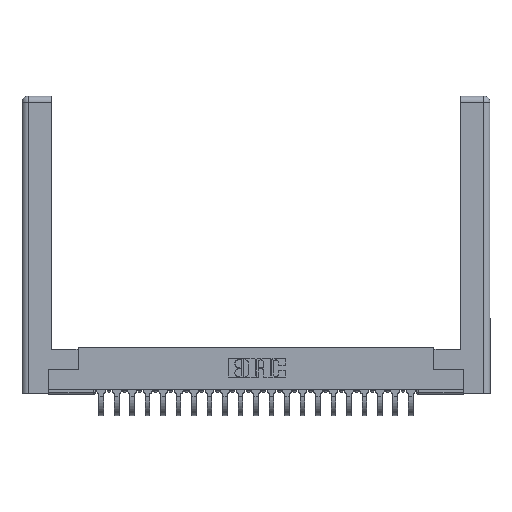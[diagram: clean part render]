
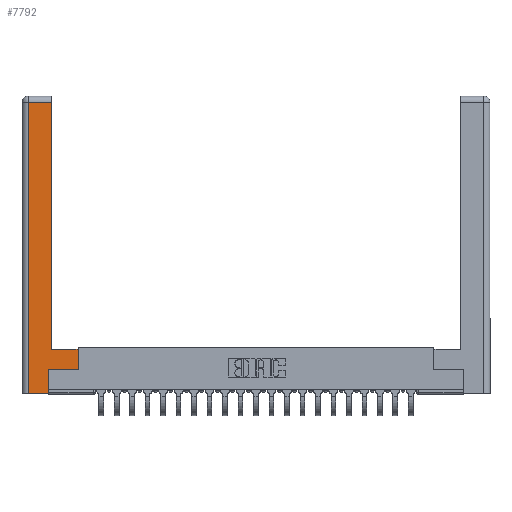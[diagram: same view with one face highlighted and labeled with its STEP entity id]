
A CAD part, top view. The second image highlights one B-rep face of the part: STEP entity #7792.
In plain terms, the highlighted planar face has unit normal (0, 0, 1).
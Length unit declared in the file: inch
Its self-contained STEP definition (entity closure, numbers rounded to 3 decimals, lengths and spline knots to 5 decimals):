
#9 = VECTOR ( 'NONE', #22567, 39.37008 ) ;
#52 = LINE ( 'NONE', #21597, #14100 ) ;
#508 = ORIENTED_EDGE ( 'NONE', *, *, #10613, .T. ) ;
#810 = EDGE_LOOP ( 'NONE', ( #508, #9398, #12760, #22565, #20387, #23384, #16623, #17363 ) ) ;
#1093 = LINE ( 'NONE', #14955, #15438 ) ;
#1332 = CARTESIAN_POINT ( 'NONE',  ( 0.565, 0.45, 0. ) ) ;
#1565 = LINE ( 'NONE', #15048, #5035 ) ;
#2089 = DIRECTION ( 'NONE',  ( 0., -1., 0. ) ) ;
#2211 = DIRECTION ( 'NONE',  ( -1., 0., 0. ) ) ;
#2525 = EDGE_CURVE ( 'NONE', #19744, #14131, #19787, .T. ) ;
#3014 = VERTEX_POINT ( 'NONE', #25304 ) ;
#3534 = DIRECTION ( 'NONE',  ( 0., 0., -1. ) ) ;
#3796 = PLANE ( 'NONE',  #17269 ) ;
#4282 = CARTESIAN_POINT ( 'NONE',  ( 0.565, 0.245, 0. ) ) ;
#4458 = CARTESIAN_POINT ( 'NONE',  ( 0.0615, 2.94, 0. ) ) ;
#4464 = CARTESIAN_POINT ( 'NONE',  ( 0.265, 0.245, 0. ) ) ;
#4528 = LINE ( 'NONE', #11958, #20076 ) ;
#5035 = VECTOR ( 'NONE', #17226, 39.37008 ) ;
#6331 = VERTEX_POINT ( 'NONE', #10448 ) ;
#6441 = EDGE_CURVE ( 'NONE', #3014, #7361, #1093, .T. ) ;
#7361 = VERTEX_POINT ( 'NONE', #15156 ) ;
#7622 = LINE ( 'NONE', #13898, #15367 ) ;
#7792 = ADVANCED_FACE ( 'NONE', ( #9799 ), #3796, .F. ) ;
#9398 = ORIENTED_EDGE ( 'NONE', *, *, #2525, .T. ) ;
#9799 = FACE_OUTER_BOUND ( 'NONE', #810, .T. ) ;
#10044 = DIRECTION ( 'NONE',  ( 0., 1., 0. ) ) ;
#10448 = CARTESIAN_POINT ( 'NONE',  ( 0.295, 0.45, 0. ) ) ;
#10587 = EDGE_CURVE ( 'NONE', #20210, #24686, #7622, .T. ) ;
#10613 = EDGE_CURVE ( 'NONE', #6331, #19744, #52, .T. ) ;
#10999 = LINE ( 'NONE', #13051, #9 ) ;
#11158 = CARTESIAN_POINT ( 'NONE',  ( 0.295, 2.94, 0. ) ) ;
#11958 = CARTESIAN_POINT ( 'NONE',  ( 0.0615, 0., 0. ) ) ;
#12526 = EDGE_CURVE ( 'NONE', #17420, #20210, #10999, .T. ) ;
#12681 = LINE ( 'NONE', #22695, #17235 ) ;
#12760 = ORIENTED_EDGE ( 'NONE', *, *, #23700, .T. ) ;
#12763 = DIRECTION ( 'NONE',  ( 1., 0., 0. ) ) ;
#13051 = CARTESIAN_POINT ( 'NONE',  ( 0.565, 0.245, 0. ) ) ;
#13898 = CARTESIAN_POINT ( 'NONE',  ( 0.565, 0.45, 0. ) ) ;
#14100 = VECTOR ( 'NONE', #21726, 39.37008 ) ;
#14131 = VERTEX_POINT ( 'NONE', #4458 ) ;
#14955 = CARTESIAN_POINT ( 'NONE',  ( 0.265, 0., 0. ) ) ;
#15048 = CARTESIAN_POINT ( 'NONE',  ( 0.295, 0.45, 0. ) ) ;
#15156 = CARTESIAN_POINT ( 'NONE',  ( 0.265, 0., 0. ) ) ;
#15343 = CARTESIAN_POINT ( 'NONE',  ( 0., 0., 0. ) ) ;
#15367 = VECTOR ( 'NONE', #10044, 39.37008 ) ;
#15438 = VECTOR ( 'NONE', #12763, 39.37008 ) ;
#16623 = ORIENTED_EDGE ( 'NONE', *, *, #10587, .T. ) ;
#17226 = DIRECTION ( 'NONE',  ( -1., 0., 0. ) ) ;
#17235 = VECTOR ( 'NONE', #20513, 39.37008 ) ;
#17269 = AXIS2_PLACEMENT_3D ( 'NONE', #15343, #3534, #23159 ) ;
#17363 = ORIENTED_EDGE ( 'NONE', *, *, #19176, .T. ) ;
#17420 = VERTEX_POINT ( 'NONE', #4464 ) ;
#19176 = EDGE_CURVE ( 'NONE', #24686, #6331, #1565, .T. ) ;
#19744 = VERTEX_POINT ( 'NONE', #11158 ) ;
#19787 = LINE ( 'NONE', #23404, #21593 ) ;
#20076 = VECTOR ( 'NONE', #2089, 39.37008 ) ;
#20210 = VERTEX_POINT ( 'NONE', #4282 ) ;
#20387 = ORIENTED_EDGE ( 'NONE', *, *, #24340, .T. ) ;
#20513 = DIRECTION ( 'NONE',  ( 0., 1., 0. ) ) ;
#21593 = VECTOR ( 'NONE', #2211, 39.37008 ) ;
#21597 = CARTESIAN_POINT ( 'NONE',  ( 0.295, 3., 0. ) ) ;
#21726 = DIRECTION ( 'NONE',  ( 0., 1., 0. ) ) ;
#22565 = ORIENTED_EDGE ( 'NONE', *, *, #6441, .T. ) ;
#22567 = DIRECTION ( 'NONE',  ( 1., 0., 0. ) ) ;
#22695 = CARTESIAN_POINT ( 'NONE',  ( 0.265, 0.245, 0. ) ) ;
#23159 = DIRECTION ( 'NONE',  ( -1., 0., 0. ) ) ;
#23384 = ORIENTED_EDGE ( 'NONE', *, *, #12526, .T. ) ;
#23404 = CARTESIAN_POINT ( 'NONE',  ( 0.0615, 2.94, 0. ) ) ;
#23700 = EDGE_CURVE ( 'NONE', #14131, #3014, #4528, .T. ) ;
#24340 = EDGE_CURVE ( 'NONE', #7361, #17420, #12681, .T. ) ;
#24686 = VERTEX_POINT ( 'NONE', #1332 ) ;
#25304 = CARTESIAN_POINT ( 'NONE',  ( 0.0615, 0., 0. ) ) ;
